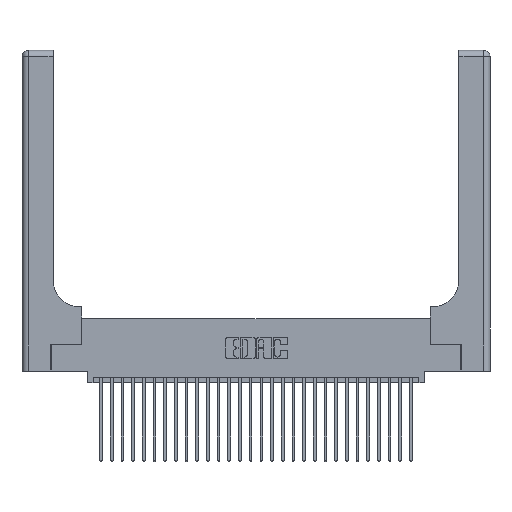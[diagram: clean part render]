
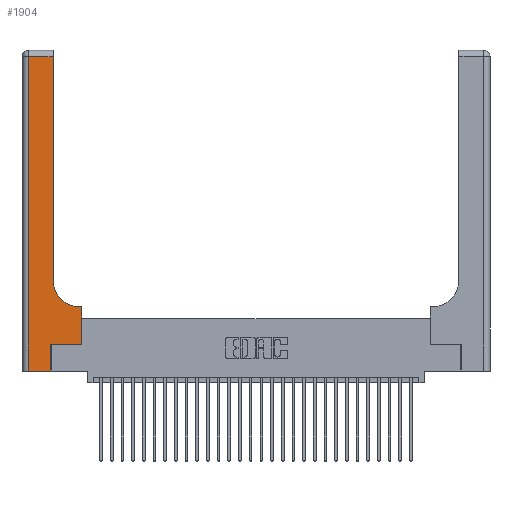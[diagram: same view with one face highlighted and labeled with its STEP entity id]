
A CAD part, top view. The second image highlights one B-rep face of the part: STEP entity #1904.
In plain terms, the highlighted planar face has unit normal (0, 0, 1).
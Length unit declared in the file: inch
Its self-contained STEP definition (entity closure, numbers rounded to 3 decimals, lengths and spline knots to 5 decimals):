
#243 = DIRECTION ( 'NONE',  ( 1., 0., 0. ) ) ;
#1126 = CARTESIAN_POINT ( 'NONE',  ( 0.06, 2.94, 0.37 ) ) ;
#1855 = CARTESIAN_POINT ( 'NONE',  ( 0.5585, 0.25, 0.37 ) ) ;
#1904 = ADVANCED_FACE ( 'NONE', ( #21870 ), #10083, .F. ) ;
#2238 = ORIENTED_EDGE ( 'NONE', *, *, #7677, .T. ) ;
#2257 = EDGE_CURVE ( 'NONE', #14955, #29818, #7501, .T. ) ;
#3343 = VECTOR ( 'NONE', #25978, 39.37008 ) ;
#3702 = CARTESIAN_POINT ( 'NONE',  ( 0.5415, 0.6, 0.37 ) ) ;
#3871 = EDGE_CURVE ( 'NONE', #10551, #13738, #15472, .T. ) ;
#4100 = LINE ( 'NONE', #17319, #28341 ) ;
#4427 = VECTOR ( 'NONE', #26994, 39.37008 ) ;
#5326 = CARTESIAN_POINT ( 'NONE',  ( 0., 3., 0.37 ) ) ;
#6881 = VECTOR ( 'NONE', #28859, 39.37008 ) ;
#6935 = VERTEX_POINT ( 'NONE', #9605 ) ;
#7459 = CARTESIAN_POINT ( 'NONE',  ( 0.269, 0.25, 0.37 ) ) ;
#7501 = LINE ( 'NONE', #1855, #25494 ) ;
#7677 = EDGE_CURVE ( 'NONE', #30143, #14955, #29080, .T. ) ;
#7844 = ORIENTED_EDGE ( 'NONE', *, *, #10881, .T. ) ;
#8124 = CARTESIAN_POINT ( 'NONE',  ( 0.269, 0., 0.37 ) ) ;
#9107 = DIRECTION ( 'NONE',  ( 0., 1., 0. ) ) ;
#9241 = CARTESIAN_POINT ( 'NONE',  ( 0.06, 3., 0.37 ) ) ;
#9605 = CARTESIAN_POINT ( 'NONE',  ( 0.2915, 0.85, 0.37 ) ) ;
#10083 = PLANE ( 'NONE',  #17140 ) ;
#10128 = CARTESIAN_POINT ( 'NONE',  ( 0.06, 0., 0.37 ) ) ;
#10376 = LINE ( 'NONE', #12719, #16612 ) ;
#10391 = ORIENTED_EDGE ( 'NONE', *, *, #19643, .T. ) ;
#10551 = VERTEX_POINT ( 'NONE', #11348 ) ;
#10881 = EDGE_CURVE ( 'NONE', #19586, #13697, #25632, .T. ) ;
#11348 = CARTESIAN_POINT ( 'NONE',  ( 0.2915, 2.94, 0.37 ) ) ;
#11370 = AXIS2_PLACEMENT_3D ( 'NONE', #28476, #14444, #243 ) ;
#11874 = ORIENTED_EDGE ( 'NONE', *, *, #3871, .T. ) ;
#12719 = CARTESIAN_POINT ( 'NONE',  ( 0.2915, 3., 0.37 ) ) ;
#13697 = VERTEX_POINT ( 'NONE', #8124 ) ;
#13738 = VERTEX_POINT ( 'NONE', #1126 ) ;
#14186 = CARTESIAN_POINT ( 'NONE',  ( 0.269, 0.25, 0.37 ) ) ;
#14433 = CIRCLE ( 'NONE', #11370, 0.25 ) ;
#14444 = DIRECTION ( 'NONE',  ( 0., 0., -1. ) ) ;
#14602 = EDGE_CURVE ( 'NONE', #13697, #30143, #26428, .T. ) ;
#14811 = DIRECTION ( 'NONE',  ( -1., 0., 0. ) ) ;
#14955 = VERTEX_POINT ( 'NONE', #17501 ) ;
#15472 = LINE ( 'NONE', #17687, #4427 ) ;
#15538 = ORIENTED_EDGE ( 'NONE', *, *, #2257, .T. ) ;
#16612 = VECTOR ( 'NONE', #22051, 39.37008 ) ;
#17067 = DIRECTION ( 'NONE',  ( 0., 0., -1. ) ) ;
#17140 = AXIS2_PLACEMENT_3D ( 'NONE', #5326, #17067, #14811 ) ;
#17319 = CARTESIAN_POINT ( 'NONE',  ( 0.2915, 0.6, 0.37 ) ) ;
#17501 = CARTESIAN_POINT ( 'NONE',  ( 0.5585, 0.25, 0.37 ) ) ;
#17687 = CARTESIAN_POINT ( 'NONE',  ( 0., 2.94, 0.37 ) ) ;
#18376 = DIRECTION ( 'NONE',  ( 0., 1., 0. ) ) ;
#19460 = EDGE_CURVE ( 'NONE', #22854, #6935, #14433, .T. ) ;
#19586 = VERTEX_POINT ( 'NONE', #10128 ) ;
#19621 = EDGE_CURVE ( 'NONE', #29818, #22854, #4100, .T. ) ;
#19643 = EDGE_CURVE ( 'NONE', #6935, #10551, #10376, .T. ) ;
#20335 = ORIENTED_EDGE ( 'NONE', *, *, #14602, .T. ) ;
#20706 = ORIENTED_EDGE ( 'NONE', *, *, #24973, .T. ) ;
#21031 = EDGE_LOOP ( 'NONE', ( #10391, #11874, #20706, #7844, #20335, #2238, #15538, #21805, #23280 ) ) ;
#21047 = DIRECTION ( 'NONE',  ( 0., -1., 0. ) ) ;
#21352 = CARTESIAN_POINT ( 'NONE',  ( 0.5585, 0.6, 0.37 ) ) ;
#21805 = ORIENTED_EDGE ( 'NONE', *, *, #19621, .T. ) ;
#21870 = FACE_OUTER_BOUND ( 'NONE', #21031, .T. ) ;
#22051 = DIRECTION ( 'NONE',  ( 0., 1., 0. ) ) ;
#22598 = VECTOR ( 'NONE', #21047, 39.37008 ) ;
#22854 = VERTEX_POINT ( 'NONE', #3702 ) ;
#23169 = CARTESIAN_POINT ( 'NONE',  ( 0.269, 0., 0.37 ) ) ;
#23280 = ORIENTED_EDGE ( 'NONE', *, *, #19460, .T. ) ;
#24973 = EDGE_CURVE ( 'NONE', #13738, #19586, #28801, .T. ) ;
#25494 = VECTOR ( 'NONE', #18376, 39.37008 ) ;
#25632 = LINE ( 'NONE', #26512, #6881 ) ;
#25978 = DIRECTION ( 'NONE',  ( 1., 0., 0. ) ) ;
#26428 = LINE ( 'NONE', #23169, #27157 ) ;
#26512 = CARTESIAN_POINT ( 'NONE',  ( 0., 0., 0.37 ) ) ;
#26739 = DIRECTION ( 'NONE',  ( -1., 0., 0. ) ) ;
#26994 = DIRECTION ( 'NONE',  ( -1., 0., 0. ) ) ;
#27157 = VECTOR ( 'NONE', #9107, 39.37008 ) ;
#28341 = VECTOR ( 'NONE', #26739, 39.37008 ) ;
#28476 = CARTESIAN_POINT ( 'NONE',  ( 0.5415, 0.85, 0.37 ) ) ;
#28801 = LINE ( 'NONE', #9241, #22598 ) ;
#28859 = DIRECTION ( 'NONE',  ( 1., 0., 0. ) ) ;
#29080 = LINE ( 'NONE', #14186, #3343 ) ;
#29818 = VERTEX_POINT ( 'NONE', #21352 ) ;
#30143 = VERTEX_POINT ( 'NONE', #7459 ) ;
